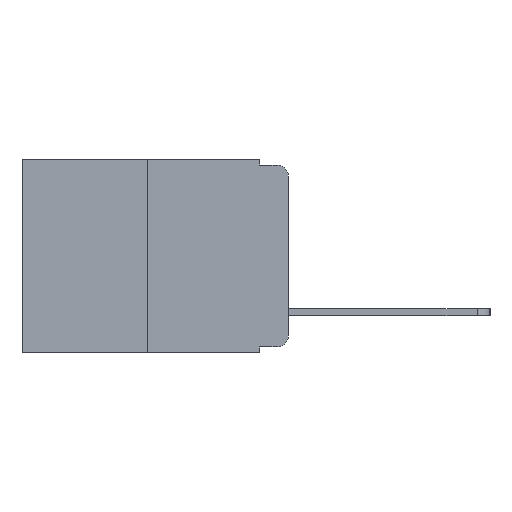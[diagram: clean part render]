
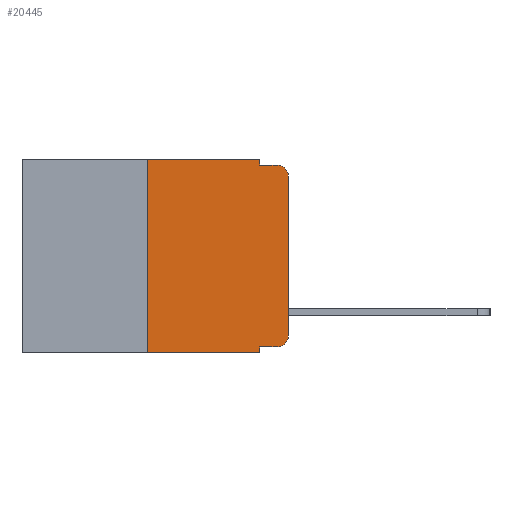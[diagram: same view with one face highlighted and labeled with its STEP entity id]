
A CAD part, left-side view. The second image highlights one B-rep face of the part: STEP entity #20445.
In plain terms, the highlighted planar face has unit normal (-1, 0, 0).
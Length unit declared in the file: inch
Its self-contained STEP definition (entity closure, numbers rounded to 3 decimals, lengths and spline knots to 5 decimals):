
#767 = AXIS2_PLACEMENT_3D ( 'NONE', #3058, #14752, #4733 ) ;
#839 = VECTOR ( 'NONE', #16117, 39.37008 ) ;
#889 = VECTOR ( 'NONE', #15764, 39.37008 ) ;
#925 = EDGE_CURVE ( 'NONE', #3253, #20025, #19529, .T. ) ;
#1032 = VECTOR ( 'NONE', #14179, 39.37008 ) ;
#1232 = EDGE_CURVE ( 'NONE', #17922, #4424, #5509, .T. ) ;
#1277 = PLANE ( 'NONE',  #767 ) ;
#1442 = VERTEX_POINT ( 'NONE', #6455 ) ;
#1796 = CARTESIAN_POINT ( 'NONE',  ( 0., 0.051, -0.333 ) ) ;
#1857 = VECTOR ( 'NONE', #21463, 39.37008 ) ;
#1922 = EDGE_LOOP ( 'NONE', ( #3092, #4792, #5469, #5669, #6284, #6377, #6423, #6751, #6824, #6911 ) ) ;
#2276 = VECTOR ( 'NONE', #15245, 39.37008 ) ;
#3058 = CARTESIAN_POINT ( 'NONE',  ( 0., 0.473, 0. ) ) ;
#3092 = ORIENTED_EDGE ( 'NONE', *, *, #4313, .T. ) ;
#3106 = AXIS2_PLACEMENT_3D ( 'NONE', #4436, #16122, #6158 ) ;
#3219 = EDGE_CURVE ( 'NONE', #12696, #20025, #14595, .T. ) ;
#3253 = VERTEX_POINT ( 'NONE', #16027 ) ;
#4313 = EDGE_CURVE ( 'NONE', #1442, #12696, #14282, .T. ) ;
#4424 = VERTEX_POINT ( 'NONE', #7808 ) ;
#4436 = CARTESIAN_POINT ( 'NONE',  ( 0., 0.02, -0.313 ) ) ;
#4476 = EDGE_CURVE ( 'NONE', #17978, #8450, #20369, .T. ) ;
#4733 = DIRECTION ( 'NONE',  ( 0., 0., -1. ) ) ;
#4792 = ORIENTED_EDGE ( 'NONE', *, *, #3219, .T. ) ;
#5469 = ORIENTED_EDGE ( 'NONE', *, *, #925, .F. ) ;
#5496 = VERTEX_POINT ( 'NONE', #12874 ) ;
#5509 = LINE ( 'NONE', #12446, #1032 ) ;
#5669 = ORIENTED_EDGE ( 'NONE', *, *, #21329, .F. ) ;
#5860 = LINE ( 'NONE', #14472, #839 ) ;
#6017 = CARTESIAN_POINT ( 'NONE',  ( 0., 0.25, 0. ) ) ;
#6034 = DIRECTION ( 'NONE',  ( 0., -1., 0. ) ) ;
#6158 = DIRECTION ( 'NONE',  ( 0., 0., -1. ) ) ;
#6284 = ORIENTED_EDGE ( 'NONE', *, *, #4476, .F. ) ;
#6377 = ORIENTED_EDGE ( 'NONE', *, *, #17019, .F. ) ;
#6423 = ORIENTED_EDGE ( 'NONE', *, *, #1232, .T. ) ;
#6455 = CARTESIAN_POINT ( 'NONE',  ( 0., 0., -0.313 ) ) ;
#6594 = CARTESIAN_POINT ( 'NONE',  ( 0., 0.051, 0. ) ) ;
#6751 = ORIENTED_EDGE ( 'NONE', *, *, #15926, .F. ) ;
#6824 = ORIENTED_EDGE ( 'NONE', *, *, #13732, .T. ) ;
#6911 = ORIENTED_EDGE ( 'NONE', *, *, #12626, .T. ) ;
#7430 = CARTESIAN_POINT ( 'NONE',  ( 0., 0., 0. ) ) ;
#7808 = CARTESIAN_POINT ( 'NONE',  ( 0., 0.051, -0.343 ) ) ;
#7983 = VECTOR ( 'NONE', #6034, 39.37008 ) ;
#8450 = VERTEX_POINT ( 'NONE', #12227 ) ;
#8643 = CARTESIAN_POINT ( 'NONE',  ( 0., 0.25, -0.343 ) ) ;
#9402 = DIRECTION ( 'NONE',  ( -1., 0., 0. ) ) ;
#9635 = LINE ( 'NONE', #11343, #17851 ) ;
#9746 = DIRECTION ( 'NONE',  ( 0., 0., -1. ) ) ;
#11343 = CARTESIAN_POINT ( 'NONE',  ( 0., 0.051, 0. ) ) ;
#11745 = LINE ( 'NONE', #6594, #2276 ) ;
#11777 = FACE_OUTER_BOUND ( 'NONE', #1922, .T. ) ;
#12178 = CIRCLE ( 'NONE', #3106, 0.02 ) ;
#12227 = CARTESIAN_POINT ( 'NONE',  ( 0., 0.051, 0. ) ) ;
#12391 = LINE ( 'NONE', #14361, #7983 ) ;
#12446 = CARTESIAN_POINT ( 'NONE',  ( 0., 0.473, -0.343 ) ) ;
#12626 = EDGE_CURVE ( 'NONE', #5496, #1442, #12178, .T. ) ;
#12696 = VERTEX_POINT ( 'NONE', #12962 ) ;
#12874 = CARTESIAN_POINT ( 'NONE',  ( 0., 0.02, -0.333 ) ) ;
#12891 = DIRECTION ( 'NONE',  ( 0., -1., 0. ) ) ;
#12909 = VERTEX_POINT ( 'NONE', #1796 ) ;
#12962 = CARTESIAN_POINT ( 'NONE',  ( 0., 0., -0.03 ) ) ;
#13395 = CARTESIAN_POINT ( 'NONE',  ( 0., 0.051, -0.01 ) ) ;
#13732 = EDGE_CURVE ( 'NONE', #12909, #5496, #12391, .T. ) ;
#14179 = DIRECTION ( 'NONE',  ( 0., -1., 0. ) ) ;
#14282 = LINE ( 'NONE', #7430, #889 ) ;
#14361 = CARTESIAN_POINT ( 'NONE',  ( 0., 0.051, -0.333 ) ) ;
#14472 = CARTESIAN_POINT ( 'NONE',  ( 0., 0.25, 0. ) ) ;
#14595 = CIRCLE ( 'NONE', #19761, 0.02 ) ;
#14752 = DIRECTION ( 'NONE',  ( 1., 0., 0. ) ) ;
#15136 = CARTESIAN_POINT ( 'NONE',  ( 0., 0.02, -0.01 ) ) ;
#15245 = DIRECTION ( 'NONE',  ( 0., 0., -1. ) ) ;
#15552 = VECTOR ( 'NONE', #12891, 39.37008 ) ;
#15764 = DIRECTION ( 'NONE',  ( 0., 0., 1. ) ) ;
#15926 = EDGE_CURVE ( 'NONE', #12909, #4424, #9635, .T. ) ;
#16027 = CARTESIAN_POINT ( 'NONE',  ( 0., 0.051, -0.01 ) ) ;
#16117 = DIRECTION ( 'NONE',  ( 0., 0., 1. ) ) ;
#16122 = DIRECTION ( 'NONE',  ( -1., 0., 0. ) ) ;
#17019 = EDGE_CURVE ( 'NONE', #17922, #17978, #5860, .T. ) ;
#17851 = VECTOR ( 'NONE', #9746, 39.37008 ) ;
#17922 = VERTEX_POINT ( 'NONE', #8643 ) ;
#17978 = VERTEX_POINT ( 'NONE', #6017 ) ;
#19232 = CARTESIAN_POINT ( 'NONE',  ( 0., 0.02, -0.03 ) ) ;
#19529 = LINE ( 'NONE', #13395, #1857 ) ;
#19761 = AXIS2_PLACEMENT_3D ( 'NONE', #19232, #9402, #20823 ) ;
#20025 = VERTEX_POINT ( 'NONE', #15136 ) ;
#20369 = LINE ( 'NONE', #20984, #15552 ) ;
#20445 = ADVANCED_FACE ( 'NONE', ( #11777 ), #1277, .F. ) ;
#20823 = DIRECTION ( 'NONE',  ( 0., 0., -1. ) ) ;
#20984 = CARTESIAN_POINT ( 'NONE',  ( 0., 0.473, 0. ) ) ;
#21329 = EDGE_CURVE ( 'NONE', #8450, #3253, #11745, .T. ) ;
#21463 = DIRECTION ( 'NONE',  ( 0., -1., 0. ) ) ;
